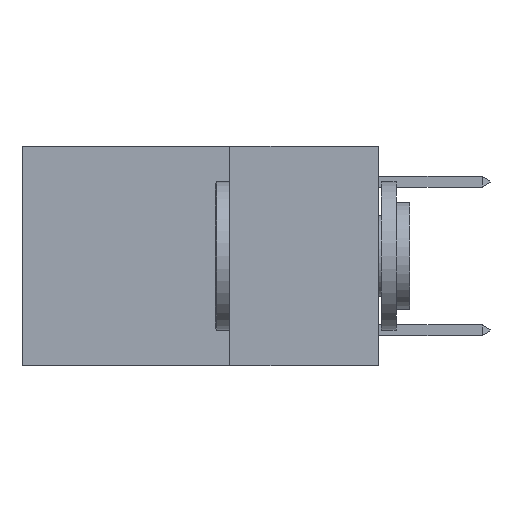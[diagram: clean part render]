
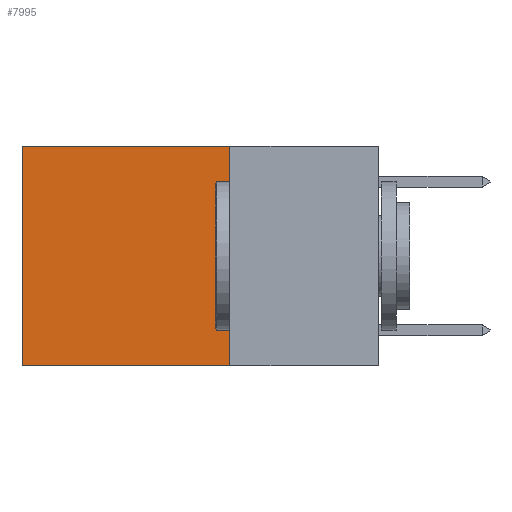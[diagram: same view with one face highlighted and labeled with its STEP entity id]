
A CAD part, left-side view. The second image highlights one B-rep face of the part: STEP entity #7995.
In plain terms, the highlighted planar face has unit normal (-1, 0, 0).
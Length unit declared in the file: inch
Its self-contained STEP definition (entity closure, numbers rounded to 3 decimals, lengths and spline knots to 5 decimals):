
#583 = CARTESIAN_POINT ( 'NONE',  ( 0.2625, 0.25, 0. ) ) ;
#2835 = VERTEX_POINT ( 'NONE', #16173 ) ;
#4298 = DIRECTION ( 'NONE',  ( 0., 0., -1. ) ) ;
#4546 = DIRECTION ( 'NONE',  ( 0., 0., -1. ) ) ;
#6037 = CARTESIAN_POINT ( 'NONE',  ( 0.2625, 0.25, 0. ) ) ;
#6435 = EDGE_CURVE ( 'NONE', #6508, #2835, #7913, .T. ) ;
#6508 = VERTEX_POINT ( 'NONE', #8430 ) ;
#7352 = CARTESIAN_POINT ( 'NONE',  ( 0.2625, 0.25, -0.37 ) ) ;
#7714 = VERTEX_POINT ( 'NONE', #14911 ) ;
#7913 = LINE ( 'NONE', #21838, #13850 ) ;
#7995 = ADVANCED_FACE ( 'NONE', ( #16269 ), #23625, .F. ) ;
#8430 = CARTESIAN_POINT ( 'NONE',  ( 0.2625, 0.6, 0. ) ) ;
#8720 = LINE ( 'NONE', #24186, #20769 ) ;
#8927 = ORIENTED_EDGE ( 'NONE', *, *, #23487, .F. ) ;
#9296 = LINE ( 'NONE', #9662, #11691 ) ;
#9662 = CARTESIAN_POINT ( 'NONE',  ( 0.2625, 0.25, 0. ) ) ;
#11691 = VECTOR ( 'NONE', #14982, 39.37008 ) ;
#13467 = VERTEX_POINT ( 'NONE', #7352 ) ;
#13850 = VECTOR ( 'NONE', #4546, 39.37008 ) ;
#14911 = CARTESIAN_POINT ( 'NONE',  ( 0.2625, 0.25, 0. ) ) ;
#14969 = ORIENTED_EDGE ( 'NONE', *, *, #24363, .T. ) ;
#14982 = DIRECTION ( 'NONE',  ( 0., 0., -1. ) ) ;
#15885 = AXIS2_PLACEMENT_3D ( 'NONE', #6037, #23498, #4298 ) ;
#16173 = CARTESIAN_POINT ( 'NONE',  ( 0.2625, 0.6, -0.37 ) ) ;
#16269 = FACE_OUTER_BOUND ( 'NONE', #20282, .T. ) ;
#17748 = DIRECTION ( 'NONE',  ( 0., 1., 0. ) ) ;
#18793 = VECTOR ( 'NONE', #21704, 39.37008 ) ;
#19664 = EDGE_CURVE ( 'NONE', #7714, #13467, #9296, .T. ) ;
#20282 = EDGE_LOOP ( 'NONE', ( #22934, #8927, #22112, #14969 ) ) ;
#20769 = VECTOR ( 'NONE', #17748, 39.37008 ) ;
#21568 = LINE ( 'NONE', #583, #18793 ) ;
#21704 = DIRECTION ( 'NONE',  ( 0., 1., 0. ) ) ;
#21838 = CARTESIAN_POINT ( 'NONE',  ( 0.2625, 0.6, 0. ) ) ;
#22112 = ORIENTED_EDGE ( 'NONE', *, *, #19664, .F. ) ;
#22934 = ORIENTED_EDGE ( 'NONE', *, *, #6435, .T. ) ;
#23487 = EDGE_CURVE ( 'NONE', #13467, #2835, #8720, .T. ) ;
#23498 = DIRECTION ( 'NONE',  ( 1., 0., 0. ) ) ;
#23625 = PLANE ( 'NONE',  #15885 ) ;
#24186 = CARTESIAN_POINT ( 'NONE',  ( 0.2625, 0.25, -0.37 ) ) ;
#24363 = EDGE_CURVE ( 'NONE', #7714, #6508, #21568, .T. ) ;
